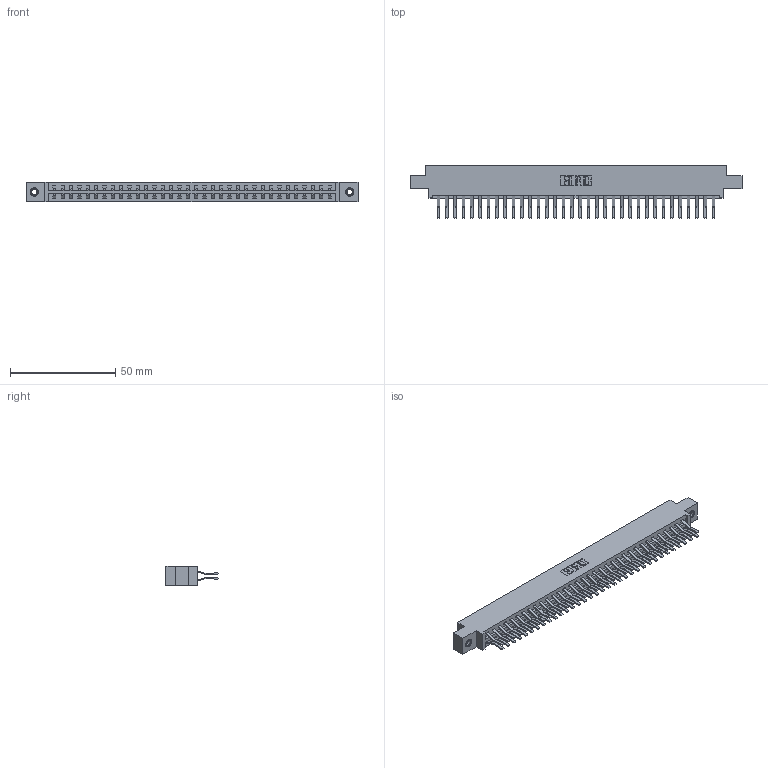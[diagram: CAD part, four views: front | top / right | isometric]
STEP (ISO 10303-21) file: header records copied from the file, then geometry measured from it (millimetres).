
FILE_DESCRIPTION (( 'STEP AP203' ), '1' );
FILE_NAME ('387-068-560-807.STEP', '2018-09-22T16:15:18', ( '' ), ( '' ), 'SwSTEP 2.0', 'SolidWorks 2016', '' );
FILE_SCHEMA (( 'CONFIG_CONTROL_DESIGN' ));
Length unit declared in the file: inch
Products named in the file (4): 337 Part_0.170 Offset - 0.156 Dia-TI; 345-292-001_560 Tail; 345-250-001_345-250-005-103; 387-068-560-807
Assembly tree (71 placements, depth 2):
  387-068-560-807
    337 Part_0.170 Offset - 0.156 Dia-TI
    345-292-001_560 Tail  x68
    345-250-001_345-250-005-103  x2
Bounding box: 157.73 x 24.78 x 9.4 mm (x, y, z)
Volume: 16831.5 mm3; surface area: 20384.1 mm2
Topology: 71 solids, 71 shells, 3986 faces, 11815 edges, 7778 vertices
Faces by surface type: plane 2690, cylinder 1280, cone 12, torus 4
Entity records: 28802 total; most frequent: CARTESIAN_POINT 4841, ORIENTED_EDGE 4770, DIRECTION 4167, EDGE_CURVE 2385, VECTOR 2233, LINE 2233, VERTEX_POINT 1584, AXIS2_PLACEMENT_3D 967
